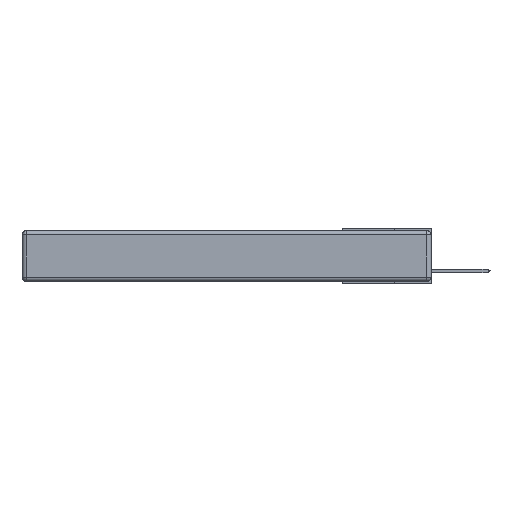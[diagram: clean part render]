
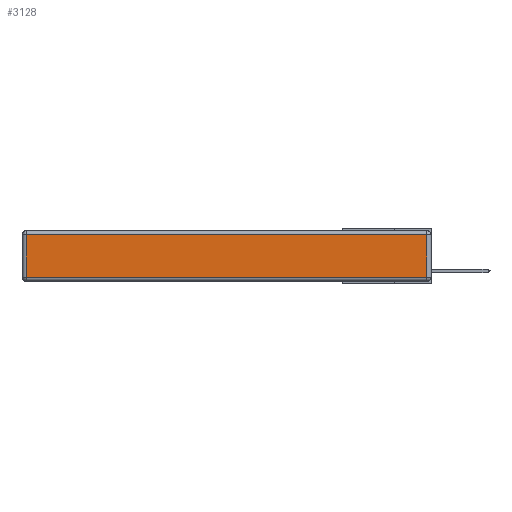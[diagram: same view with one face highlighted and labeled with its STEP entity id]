
A CAD part, left-side view. The second image highlights one B-rep face of the part: STEP entity #3128.
In plain terms, the highlighted planar face has unit normal (-1, 0, 0).
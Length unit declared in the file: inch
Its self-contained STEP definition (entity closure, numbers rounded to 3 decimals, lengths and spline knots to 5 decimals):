
#1039 = VECTOR ( 'NONE', #9781, 39.37008 ) ;
#3128 = ADVANCED_FACE ( 'NONE', ( #24546 ), #13177, .T. ) ;
#3411 = EDGE_CURVE ( 'NONE', #14817, #8995, #15177, .T. ) ;
#4202 = LINE ( 'NONE', #16996, #26059 ) ;
#4811 = EDGE_CURVE ( 'NONE', #12565, #14817, #4202, .T. ) ;
#5873 = EDGE_LOOP ( 'NONE', ( #9541, #12061, #17006, #24184 ) ) ;
#8995 = VERTEX_POINT ( 'NONE', #19149 ) ;
#9167 = VECTOR ( 'NONE', #19098, 39.37008 ) ;
#9541 = ORIENTED_EDGE ( 'NONE', *, *, #23808, .T. ) ;
#9645 = AXIS2_PLACEMENT_3D ( 'NONE', #14883, #16971, #10849 ) ;
#9781 = DIRECTION ( 'NONE',  ( 0., 1., 0. ) ) ;
#10393 = LINE ( 'NONE', #23427, #22271 ) ;
#10849 = DIRECTION ( 'NONE',  ( 0., 0., 1. ) ) ;
#11921 = CARTESIAN_POINT ( 'NONE',  ( 0., 2.75, -0.03 ) ) ;
#12061 = ORIENTED_EDGE ( 'NONE', *, *, #4811, .T. ) ;
#12565 = VERTEX_POINT ( 'NONE', #25169 ) ;
#13177 = PLANE ( 'NONE',  #9645 ) ;
#13673 = VERTEX_POINT ( 'NONE', #21285 ) ;
#14817 = VERTEX_POINT ( 'NONE', #24927 ) ;
#14883 = CARTESIAN_POINT ( 'NONE',  ( 0., 0., -0.343 ) ) ;
#15177 = LINE ( 'NONE', #11921, #1039 ) ;
#16971 = DIRECTION ( 'NONE',  ( -1., 0., 0. ) ) ;
#16996 = CARTESIAN_POINT ( 'NONE',  ( 0., 0.03, -0.343 ) ) ;
#17006 = ORIENTED_EDGE ( 'NONE', *, *, #3411, .T. ) ;
#17767 = DIRECTION ( 'NONE',  ( 0., -1., 0. ) ) ;
#18790 = LINE ( 'NONE', #25229, #9167 ) ;
#19098 = DIRECTION ( 'NONE',  ( 0., 0., -1. ) ) ;
#19149 = CARTESIAN_POINT ( 'NONE',  ( 0., 2.72, -0.03 ) ) ;
#21285 = CARTESIAN_POINT ( 'NONE',  ( 0., 2.72, -0.313 ) ) ;
#22271 = VECTOR ( 'NONE', #17767, 39.37008 ) ;
#22383 = EDGE_CURVE ( 'NONE', #8995, #13673, #18790, .T. ) ;
#23427 = CARTESIAN_POINT ( 'NONE',  ( 0., 0., -0.313 ) ) ;
#23808 = EDGE_CURVE ( 'NONE', #13673, #12565, #10393, .T. ) ;
#24184 = ORIENTED_EDGE ( 'NONE', *, *, #22383, .T. ) ;
#24546 = FACE_OUTER_BOUND ( 'NONE', #5873, .T. ) ;
#24927 = CARTESIAN_POINT ( 'NONE',  ( 0., 0.03, -0.03 ) ) ;
#25169 = CARTESIAN_POINT ( 'NONE',  ( 0., 0.03, -0.313 ) ) ;
#25229 = CARTESIAN_POINT ( 'NONE',  ( 0., 2.72, -0.343 ) ) ;
#25530 = DIRECTION ( 'NONE',  ( 0., 0., 1. ) ) ;
#26059 = VECTOR ( 'NONE', #25530, 39.37008 ) ;
